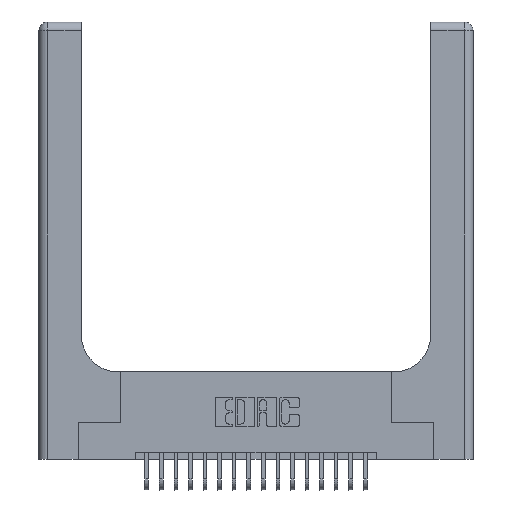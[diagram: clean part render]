
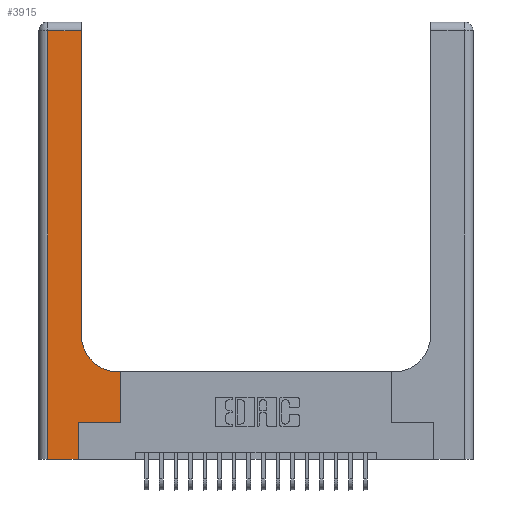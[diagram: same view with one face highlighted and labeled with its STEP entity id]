
A CAD part, top view. The second image highlights one B-rep face of the part: STEP entity #3915.
In plain terms, the highlighted planar face has unit normal (0, 0, 1).
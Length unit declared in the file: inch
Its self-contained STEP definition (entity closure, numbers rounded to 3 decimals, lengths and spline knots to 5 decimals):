
#336 = LINE ( 'NONE', #22204, #9485 ) ;
#758 = DIRECTION ( 'NONE',  ( 0., 1., 0. ) ) ;
#1327 = DIRECTION ( 'NONE',  ( 0., 0., -1. ) ) ;
#1690 = VECTOR ( 'NONE', #18949, 39.37008 ) ;
#1757 = CIRCLE ( 'NONE', #4407, 0.25 ) ;
#2281 = LINE ( 'NONE', #13857, #1690 ) ;
#2466 = CARTESIAN_POINT ( 'NONE',  ( 0.5585, 0.25, 0.37 ) ) ;
#2982 = LINE ( 'NONE', #21873, #12418 ) ;
#3915 = ADVANCED_FACE ( 'NONE', ( #17657 ), #17264, .F. ) ;
#4141 = VECTOR ( 'NONE', #14712, 39.37008 ) ;
#4407 = AXIS2_PLACEMENT_3D ( 'NONE', #12080, #1327, #13831 ) ;
#4594 = CARTESIAN_POINT ( 'NONE',  ( 0., 2.94, 0.37 ) ) ;
#4708 = EDGE_LOOP ( 'NONE', ( #13790, #13980, #14059, #14526, #14738, #14827, #15108, #15342, #15847 ) ) ;
#5176 = CARTESIAN_POINT ( 'NONE',  ( 0.06, 0., 0.37 ) ) ;
#5478 = VERTEX_POINT ( 'NONE', #2466 ) ;
#5942 = CARTESIAN_POINT ( 'NONE',  ( 0.5585, 0.25, 0.37 ) ) ;
#6525 = CARTESIAN_POINT ( 'NONE',  ( 0.5585, 0.6, 0.37 ) ) ;
#6845 = DIRECTION ( 'NONE',  ( 0., 0., -1. ) ) ;
#6892 = EDGE_CURVE ( 'NONE', #13864, #11660, #1757, .T. ) ;
#6932 = VECTOR ( 'NONE', #12234, 39.37008 ) ;
#7202 = EDGE_CURVE ( 'NONE', #11937, #10104, #18040, .T. ) ;
#7417 = VECTOR ( 'NONE', #19590, 39.37008 ) ;
#7503 = LINE ( 'NONE', #22564, #6932 ) ;
#8163 = DIRECTION ( 'NONE',  ( 1., 0., 0. ) ) ;
#8451 = EDGE_CURVE ( 'NONE', #5478, #14997, #16461, .T. ) ;
#9485 = VECTOR ( 'NONE', #15358, 39.37008 ) ;
#9932 = CARTESIAN_POINT ( 'NONE',  ( 0.269, 0.25, 0.37 ) ) ;
#10104 = VERTEX_POINT ( 'NONE', #20679 ) ;
#10199 = AXIS2_PLACEMENT_3D ( 'NONE', #12050, #6845, #18968 ) ;
#10366 = EDGE_CURVE ( 'NONE', #14997, #13864, #12600, .T. ) ;
#11380 = CARTESIAN_POINT ( 'NONE',  ( 0.2915, 0.85, 0.37 ) ) ;
#11660 = VERTEX_POINT ( 'NONE', #11380 ) ;
#11937 = VERTEX_POINT ( 'NONE', #15514 ) ;
#12050 = CARTESIAN_POINT ( 'NONE',  ( 0., 3., 0.37 ) ) ;
#12080 = CARTESIAN_POINT ( 'NONE',  ( 0.5415, 0.85, 0.37 ) ) ;
#12171 = VERTEX_POINT ( 'NONE', #19860 ) ;
#12234 = DIRECTION ( 'NONE',  ( 0., 1., 0. ) ) ;
#12418 = VECTOR ( 'NONE', #758, 39.37008 ) ;
#12600 = LINE ( 'NONE', #12692, #7417 ) ;
#12646 = LINE ( 'NONE', #9932, #20720 ) ;
#12692 = CARTESIAN_POINT ( 'NONE',  ( 0.2915, 0.6, 0.37 ) ) ;
#13790 = ORIENTED_EDGE ( 'NONE', *, *, #15383, .T. ) ;
#13831 = DIRECTION ( 'NONE',  ( 1., 0., 0. ) ) ;
#13857 = CARTESIAN_POINT ( 'NONE',  ( 0., 0., 0.37 ) ) ;
#13864 = VERTEX_POINT ( 'NONE', #17637 ) ;
#13980 = ORIENTED_EDGE ( 'NONE', *, *, #7202, .T. ) ;
#14059 = ORIENTED_EDGE ( 'NONE', *, *, #20830, .T. ) ;
#14526 = ORIENTED_EDGE ( 'NONE', *, *, #17314, .T. ) ;
#14712 = DIRECTION ( 'NONE',  ( 0., 1., 0. ) ) ;
#14738 = ORIENTED_EDGE ( 'NONE', *, *, #15650, .T. ) ;
#14827 = ORIENTED_EDGE ( 'NONE', *, *, #16573, .T. ) ;
#14997 = VERTEX_POINT ( 'NONE', #6525 ) ;
#15080 = DIRECTION ( 'NONE',  ( -1., 0., 0. ) ) ;
#15108 = ORIENTED_EDGE ( 'NONE', *, *, #8451, .T. ) ;
#15342 = ORIENTED_EDGE ( 'NONE', *, *, #10366, .T. ) ;
#15358 = DIRECTION ( 'NONE',  ( 0., -1., 0. ) ) ;
#15383 = EDGE_CURVE ( 'NONE', #11660, #11937, #2982, .T. ) ;
#15514 = CARTESIAN_POINT ( 'NONE',  ( 0.2915, 2.94, 0.37 ) ) ;
#15650 = EDGE_CURVE ( 'NONE', #12171, #22444, #7503, .T. ) ;
#15847 = ORIENTED_EDGE ( 'NONE', *, *, #6892, .T. ) ;
#16461 = LINE ( 'NONE', #5942, #4141 ) ;
#16573 = EDGE_CURVE ( 'NONE', #22444, #5478, #12646, .T. ) ;
#17264 = PLANE ( 'NONE',  #10199 ) ;
#17314 = EDGE_CURVE ( 'NONE', #19264, #12171, #2281, .T. ) ;
#17637 = CARTESIAN_POINT ( 'NONE',  ( 0.5415, 0.6, 0.37 ) ) ;
#17657 = FACE_OUTER_BOUND ( 'NONE', #4708, .T. ) ;
#18040 = LINE ( 'NONE', #4594, #22061 ) ;
#18949 = DIRECTION ( 'NONE',  ( 1., 0., 0. ) ) ;
#18968 = DIRECTION ( 'NONE',  ( -1., 0., 0. ) ) ;
#19264 = VERTEX_POINT ( 'NONE', #5176 ) ;
#19590 = DIRECTION ( 'NONE',  ( -1., 0., 0. ) ) ;
#19860 = CARTESIAN_POINT ( 'NONE',  ( 0.269, 0., 0.37 ) ) ;
#20679 = CARTESIAN_POINT ( 'NONE',  ( 0.06, 2.94, 0.37 ) ) ;
#20720 = VECTOR ( 'NONE', #8163, 39.37008 ) ;
#20830 = EDGE_CURVE ( 'NONE', #10104, #19264, #336, .T. ) ;
#21873 = CARTESIAN_POINT ( 'NONE',  ( 0.2915, 3., 0.37 ) ) ;
#21981 = CARTESIAN_POINT ( 'NONE',  ( 0.269, 0.25, 0.37 ) ) ;
#22061 = VECTOR ( 'NONE', #15080, 39.37008 ) ;
#22204 = CARTESIAN_POINT ( 'NONE',  ( 0.06, 3., 0.37 ) ) ;
#22444 = VERTEX_POINT ( 'NONE', #21981 ) ;
#22564 = CARTESIAN_POINT ( 'NONE',  ( 0.269, 0., 0.37 ) ) ;
